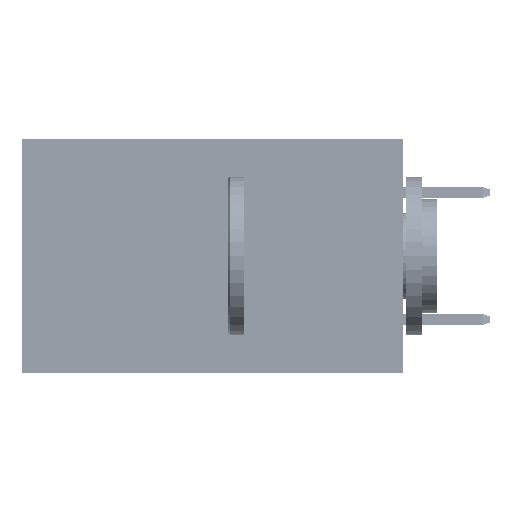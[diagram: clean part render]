
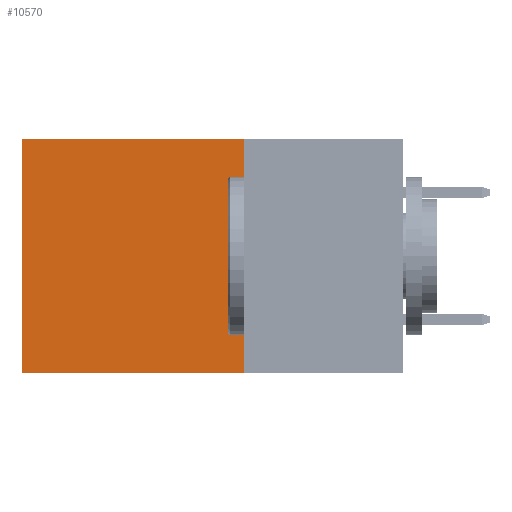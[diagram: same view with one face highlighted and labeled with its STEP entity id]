
A CAD part, left-side view. The second image highlights one B-rep face of the part: STEP entity #10570.
In plain terms, the highlighted planar face has unit normal (-1, 0, 0).
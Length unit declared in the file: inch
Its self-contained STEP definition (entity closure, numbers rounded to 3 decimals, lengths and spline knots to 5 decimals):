
#607 = VERTEX_POINT ( 'NONE', #18455 ) ;
#2744 = DIRECTION ( 'NONE',  ( 0., 1., 0. ) ) ;
#3254 = CARTESIAN_POINT ( 'NONE',  ( 0.2875, 0.25, -0.37 ) ) ;
#3363 = EDGE_CURVE ( 'NONE', #24209, #607, #28780, .T. ) ;
#6859 = ORIENTED_EDGE ( 'NONE', *, *, #29758, .F. ) ;
#7246 = LINE ( 'NONE', #3254, #29849 ) ;
#7771 = DIRECTION ( 'NONE',  ( 0., 0., -1. ) ) ;
#10570 = ADVANCED_FACE ( 'NONE', ( #39062 ), #51593, .F. ) ;
#13139 = CARTESIAN_POINT ( 'NONE',  ( 0.2875, 0.25, -0.37 ) ) ;
#13838 = VECTOR ( 'NONE', #18725, 39.37008 ) ;
#15138 = CARTESIAN_POINT ( 'NONE',  ( 0.2875, 0.25, 0. ) ) ;
#16291 = VERTEX_POINT ( 'NONE', #27935 ) ;
#17470 = DIRECTION ( 'NONE',  ( 0., 1., 0. ) ) ;
#17724 = CARTESIAN_POINT ( 'NONE',  ( 0.2875, 0.25, 0. ) ) ;
#18455 = CARTESIAN_POINT ( 'NONE',  ( 0.2875, 0.6, -0.37 ) ) ;
#18725 = DIRECTION ( 'NONE',  ( 0., 0., -1. ) ) ;
#20063 = ORIENTED_EDGE ( 'NONE', *, *, #49602, .T. ) ;
#21975 = LINE ( 'NONE', #17724, #40464 ) ;
#22464 = CARTESIAN_POINT ( 'NONE',  ( 0.2875, 0.25, 0. ) ) ;
#22623 = VECTOR ( 'NONE', #7771, 39.37008 ) ;
#23754 = AXIS2_PLACEMENT_3D ( 'NONE', #15138, #31369, #39577 ) ;
#24209 = VERTEX_POINT ( 'NONE', #30916 ) ;
#27935 = CARTESIAN_POINT ( 'NONE',  ( 0.2875, 0.25, 0. ) ) ;
#27997 = CARTESIAN_POINT ( 'NONE',  ( 0.2875, 0.6, 0. ) ) ;
#28780 = LINE ( 'NONE', #27997, #22623 ) ;
#29758 = EDGE_CURVE ( 'NONE', #16291, #38311, #50424, .T. ) ;
#29849 = VECTOR ( 'NONE', #2744, 39.37008 ) ;
#30916 = CARTESIAN_POINT ( 'NONE',  ( 0.2875, 0.6, 0. ) ) ;
#31369 = DIRECTION ( 'NONE',  ( 1., 0., 0. ) ) ;
#38311 = VERTEX_POINT ( 'NONE', #13139 ) ;
#39062 = FACE_OUTER_BOUND ( 'NONE', #46007, .T. ) ;
#39577 = DIRECTION ( 'NONE',  ( 0., 0., -1. ) ) ;
#40464 = VECTOR ( 'NONE', #17470, 39.37008 ) ;
#43279 = EDGE_CURVE ( 'NONE', #38311, #607, #7246, .T. ) ;
#44439 = ORIENTED_EDGE ( 'NONE', *, *, #43279, .F. ) ;
#46007 = EDGE_LOOP ( 'NONE', ( #46486, #44439, #6859, #20063 ) ) ;
#46486 = ORIENTED_EDGE ( 'NONE', *, *, #3363, .T. ) ;
#49602 = EDGE_CURVE ( 'NONE', #16291, #24209, #21975, .T. ) ;
#50424 = LINE ( 'NONE', #22464, #13838 ) ;
#51593 = PLANE ( 'NONE',  #23754 ) ;
